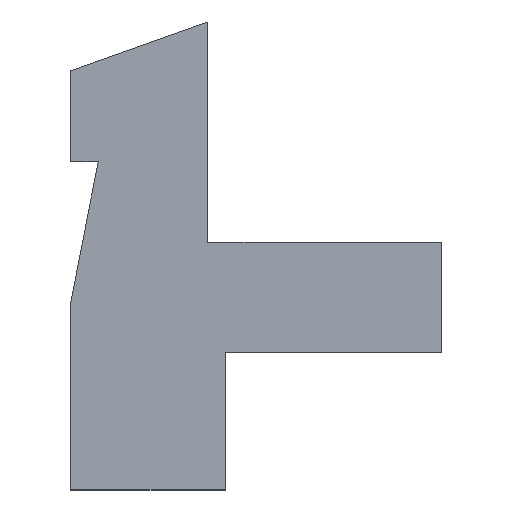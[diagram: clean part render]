
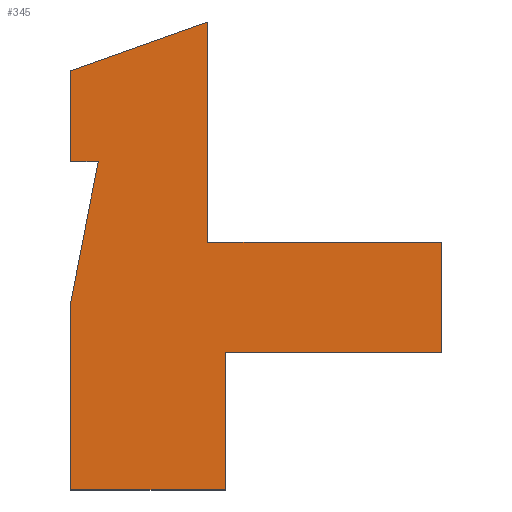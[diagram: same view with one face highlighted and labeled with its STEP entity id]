
A CAD part, top view. The second image highlights one B-rep face of the part: STEP entity #345.
In plain terms, the highlighted planar face has unit normal (0, 0, 1).
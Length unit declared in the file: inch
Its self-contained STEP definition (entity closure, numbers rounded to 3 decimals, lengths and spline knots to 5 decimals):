
#31=FACE_OUTER_BOUND('',#51,.T.);
#51=EDGE_LOOP('',(#274,#275,#276,#277,#278,#279,#280,#281,#282,#283,#284,
#285,#286,#287));
#62=LINE('',#485,#106);
#68=LINE('',#504,#112);
#71=LINE('',#511,#115);
#76=LINE('',#520,#120);
#79=LINE('',#526,#123);
#89=LINE('',#545,#133);
#91=LINE('',#548,#135);
#92=LINE('',#549,#136);
#93=LINE('',#551,#137);
#94=LINE('',#553,#138);
#95=LINE('',#555,#139);
#96=LINE('',#557,#140);
#97=LINE('',#559,#141);
#98=LINE('',#560,#142);
#106=VECTOR('',#395,0.3937);
#112=VECTOR('',#413,39.37008);
#115=VECTOR('',#418,39.37008);
#120=VECTOR('',#425,39.37008);
#123=VECTOR('',#430,39.37008);
#133=VECTOR('',#444,39.37008);
#135=VECTOR('',#448,39.37008);
#136=VECTOR('',#449,39.37008);
#137=VECTOR('',#450,39.37008);
#138=VECTOR('',#451,39.37008);
#139=VECTOR('',#452,39.37008);
#140=VECTOR('',#453,39.37008);
#141=VECTOR('',#454,39.37008);
#142=VECTOR('',#455,39.37008);
#150=VERTEX_POINT('',#482);
#151=VERTEX_POINT('',#484);
#157=VERTEX_POINT('',#501);
#158=VERTEX_POINT('',#503);
#159=VERTEX_POINT('',#507);
#161=VERTEX_POINT('',#510);
#164=VERTEX_POINT('',#518);
#166=VERTEX_POINT('',#524);
#173=VERTEX_POINT('',#544);
#174=VERTEX_POINT('',#550);
#175=VERTEX_POINT('',#552);
#176=VERTEX_POINT('',#554);
#177=VERTEX_POINT('',#556);
#178=VERTEX_POINT('',#558);
#181=EDGE_CURVE('',#150,#151,#62,.T.);
#190=EDGE_CURVE('',#158,#157,#68,.T.);
#193=EDGE_CURVE('',#159,#161,#71,.T.);
#198=EDGE_CURVE('',#159,#164,#76,.T.);
#201=EDGE_CURVE('',#164,#166,#79,.T.);
#211=EDGE_CURVE('',#161,#173,#89,.T.);
#213=EDGE_CURVE('',#166,#158,#91,.T.);
#214=EDGE_CURVE('',#157,#151,#92,.T.);
#215=EDGE_CURVE('',#174,#150,#93,.T.);
#216=EDGE_CURVE('',#174,#175,#94,.T.);
#217=EDGE_CURVE('',#175,#176,#95,.T.);
#218=EDGE_CURVE('',#176,#177,#96,.T.);
#219=EDGE_CURVE('',#177,#178,#97,.T.);
#220=EDGE_CURVE('',#178,#173,#98,.T.);
#274=ORIENTED_EDGE('',*,*,#193,.F.);
#275=ORIENTED_EDGE('',*,*,#198,.T.);
#276=ORIENTED_EDGE('',*,*,#201,.T.);
#277=ORIENTED_EDGE('',*,*,#213,.T.);
#278=ORIENTED_EDGE('',*,*,#190,.T.);
#279=ORIENTED_EDGE('',*,*,#214,.T.);
#280=ORIENTED_EDGE('',*,*,#181,.F.);
#281=ORIENTED_EDGE('',*,*,#215,.F.);
#282=ORIENTED_EDGE('',*,*,#216,.T.);
#283=ORIENTED_EDGE('',*,*,#217,.T.);
#284=ORIENTED_EDGE('',*,*,#218,.T.);
#285=ORIENTED_EDGE('',*,*,#219,.T.);
#286=ORIENTED_EDGE('',*,*,#220,.T.);
#287=ORIENTED_EDGE('',*,*,#211,.F.);
#327=PLANE('',#380);
#345=ADVANCED_FACE('',(#31),#327,.T.);
#380=AXIS2_PLACEMENT_3D('',#547,#446,#447);
#395=DIRECTION('',(0.942,0.335,0.));
#413=DIRECTION('',(-1.,0.,0.));
#418=DIRECTION('',(-1.,0.,0.));
#425=DIRECTION('',(0.,1.,0.));
#430=DIRECTION('',(1.,0.,0.));
#444=DIRECTION('',(0.,1.,0.));
#446=DIRECTION('center_axis',(0.,0.,1.));
#447=DIRECTION('ref_axis',(-1.,0.,0.));
#448=DIRECTION('',(0.,1.,0.));
#449=DIRECTION('',(0.,1.,0.));
#450=DIRECTION('',(0.,1.,0.));
#451=DIRECTION('',(1.,0.,0.));
#452=DIRECTION('',(-0.191,-0.982,0.));
#453=DIRECTION('',(1.,0.,0.));
#454=DIRECTION('',(-0.193,-0.981,0.));
#455=DIRECTION('',(-0.191,-0.982,0.));
#482=CARTESIAN_POINT('',(-0.99753,0.46548,0.23622));
#484=CARTESIAN_POINT('',(-0.80068,0.53553,0.23622));
#485=CARTESIAN_POINT('',(-0.99753,0.46548,0.23622));
#501=CARTESIAN_POINT('',(-0.80068,0.21992,0.23622));
#503=CARTESIAN_POINT('',(-0.46604,0.21992,0.23622));
#504=CARTESIAN_POINT('',(-0.63336,0.21992,0.23622));
#507=CARTESIAN_POINT('',(-0.77559,-0.13441,0.23622));
#510=CARTESIAN_POINT('',(-0.99753,-0.13441,0.23622));
#511=CARTESIAN_POINT('',(-0.73178,-0.13441,0.23622));
#518=CARTESIAN_POINT('',(-0.77559,0.06244,0.23622));
#520=CARTESIAN_POINT('',(-0.77559,-0.80126,0.23622));
#524=CARTESIAN_POINT('',(-0.46604,0.06244,0.23622));
#526=CARTESIAN_POINT('',(-0.7709,0.06244,0.23622));
#544=CARTESIAN_POINT('',(-0.99753,0.13146,0.23622));
#545=CARTESIAN_POINT('',(-0.99753,-0.33126,0.23622));
#547=CARTESIAN_POINT('Origin',(-0.46604,-0.33126,0.23622));
#548=CARTESIAN_POINT('',(-0.46604,-0.33126,0.23622));
#549=CARTESIAN_POINT('',(-0.80068,0.07228,0.23622));
#550=CARTESIAN_POINT('',(-0.99753,0.33629,0.23622));
#551=CARTESIAN_POINT('',(-0.99753,-0.33126,0.23622));
#552=CARTESIAN_POINT('',(-0.95772,0.33629,0.23622));
#553=CARTESIAN_POINT('',(-0.99753,0.33629,0.23622));
#554=CARTESIAN_POINT('',(-0.9646,0.30091,0.23622));
#555=CARTESIAN_POINT('',(-0.95772,0.33629,0.23622));
#556=CARTESIAN_POINT('',(-0.96449,0.30091,0.23622));
#557=CARTESIAN_POINT('',(-1.10301,0.30091,0.23622));
#558=CARTESIAN_POINT('',(-0.97317,0.25679,0.23622));
#559=CARTESIAN_POINT('',(-0.96449,0.30091,0.23622));
#560=CARTESIAN_POINT('',(-0.95772,0.33629,0.23622));
